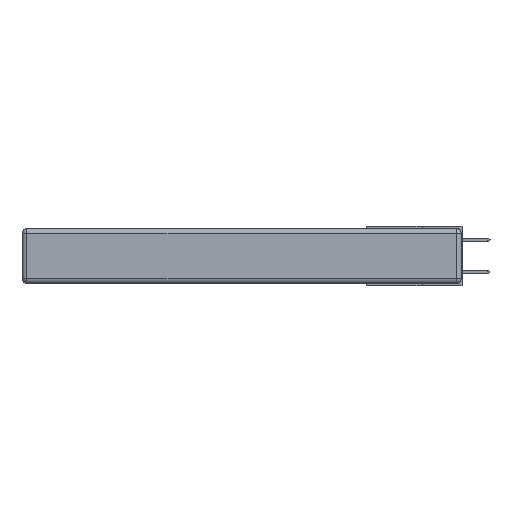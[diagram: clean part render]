
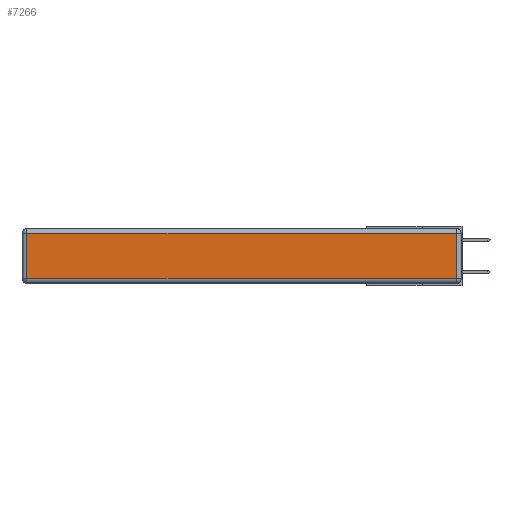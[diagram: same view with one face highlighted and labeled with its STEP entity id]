
A CAD part, left-side view. The second image highlights one B-rep face of the part: STEP entity #7266.
In plain terms, the highlighted planar face has unit normal (-1, 0, 0).
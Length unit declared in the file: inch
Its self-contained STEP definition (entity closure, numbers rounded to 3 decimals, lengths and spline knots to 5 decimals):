
#932 = LINE ( 'NONE', #18513, #16403 ) ;
#1265 = LINE ( 'NONE', #2656, #9992 ) ;
#1327 = DIRECTION ( 'NONE',  ( 0., 0., 1. ) ) ;
#1519 = EDGE_CURVE ( 'NONE', #12795, #11401, #1265, .T. ) ;
#2271 = CARTESIAN_POINT ( 'NONE',  ( 0., 2.72, -0.03 ) ) ;
#2333 = LINE ( 'NONE', #21746, #4269 ) ;
#2432 = DIRECTION ( 'NONE',  ( 0., 1., 0. ) ) ;
#2656 = CARTESIAN_POINT ( 'NONE',  ( 0., 2.75, -0.03 ) ) ;
#2899 = ORIENTED_EDGE ( 'NONE', *, *, #10272, .T. ) ;
#4269 = VECTOR ( 'NONE', #14568, 39.37008 ) ;
#4685 = CARTESIAN_POINT ( 'NONE',  ( 0., 0.03, -0.03 ) ) ;
#5070 = DIRECTION ( 'NONE',  ( 0., 0., -1. ) ) ;
#5130 = EDGE_LOOP ( 'NONE', ( #9122, #18423, #14321, #2899 ) ) ;
#5572 = VECTOR ( 'NONE', #5070, 39.37008 ) ;
#6566 = FACE_OUTER_BOUND ( 'NONE', #5130, .T. ) ;
#7266 = ADVANCED_FACE ( 'NONE', ( #6566 ), #15153, .T. ) ;
#9122 = ORIENTED_EDGE ( 'NONE', *, *, #14006, .T. ) ;
#9992 = VECTOR ( 'NONE', #2432, 39.37008 ) ;
#10272 = EDGE_CURVE ( 'NONE', #11401, #13478, #19143, .T. ) ;
#11401 = VERTEX_POINT ( 'NONE', #2271 ) ;
#11835 = DIRECTION ( 'NONE',  ( -1., 0., 0. ) ) ;
#12795 = VERTEX_POINT ( 'NONE', #4685 ) ;
#13272 = CARTESIAN_POINT ( 'NONE',  ( 0., 0., -0.343 ) ) ;
#13478 = VERTEX_POINT ( 'NONE', #15044 ) ;
#14006 = EDGE_CURVE ( 'NONE', #13478, #22111, #932, .T. ) ;
#14321 = ORIENTED_EDGE ( 'NONE', *, *, #1519, .T. ) ;
#14568 = DIRECTION ( 'NONE',  ( 0., 0., 1. ) ) ;
#15044 = CARTESIAN_POINT ( 'NONE',  ( 0., 2.72, -0.313 ) ) ;
#15153 = PLANE ( 'NONE',  #19019 ) ;
#16403 = VECTOR ( 'NONE', #18435, 39.37008 ) ;
#17924 = EDGE_CURVE ( 'NONE', #22111, #12795, #2333, .T. ) ;
#18423 = ORIENTED_EDGE ( 'NONE', *, *, #17924, .T. ) ;
#18435 = DIRECTION ( 'NONE',  ( 0., -1., 0. ) ) ;
#18513 = CARTESIAN_POINT ( 'NONE',  ( 0., 0., -0.313 ) ) ;
#18736 = CARTESIAN_POINT ( 'NONE',  ( 0., 0.03, -0.313 ) ) ;
#19019 = AXIS2_PLACEMENT_3D ( 'NONE', #13272, #11835, #1327 ) ;
#19143 = LINE ( 'NONE', #20388, #5572 ) ;
#20388 = CARTESIAN_POINT ( 'NONE',  ( 0., 2.72, -0.343 ) ) ;
#21746 = CARTESIAN_POINT ( 'NONE',  ( 0., 0.03, -0.343 ) ) ;
#22111 = VERTEX_POINT ( 'NONE', #18736 ) ;
